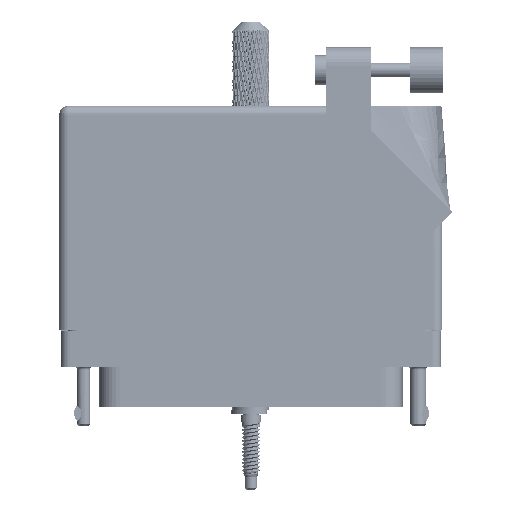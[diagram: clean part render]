
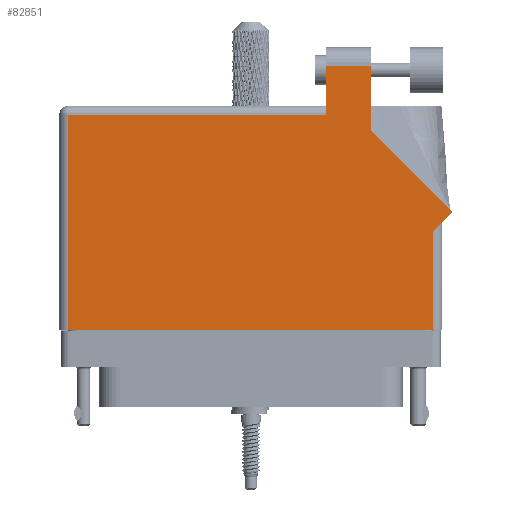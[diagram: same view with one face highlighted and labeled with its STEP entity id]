
A CAD part, front view. The second image highlights one B-rep face of the part: STEP entity #82851.
In plain terms, the highlighted face is planar.
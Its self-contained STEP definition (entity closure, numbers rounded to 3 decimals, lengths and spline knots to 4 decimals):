
#485 = EDGE_LOOP ( 'NONE', ( #99890, #19792, #51032, #76020, #92386, #72344, #46779, #94173, #6920 ) ) ;
#732 = EDGE_CURVE ( 'NONE', #107216, #65128, #65377, .T. ) ;
#1587 = VERTEX_POINT ( 'NONE', #102448 ) ;
#4742 = CARTESIAN_POINT ( 'NONE',  ( 0.82, 1.705, 0.455 ) ) ;
#5393 = LINE ( 'NONE', #80090, #112568 ) ;
#5544 = PLANE ( 'NONE',  #17887 ) ;
#5785 = VERTEX_POINT ( 'NONE', #7285 ) ;
#6920 = ORIENTED_EDGE ( 'NONE', *, *, #72758, .T. ) ;
#7285 = CARTESIAN_POINT ( 'NONE',  ( -1.244, 1.368, 0.455 ) ) ;
#10316 = EDGE_CURVE ( 'NONE', #88586, #28034, #113640, .T. ) ;
#12041 = CARTESIAN_POINT ( 'NONE',  ( 0.513, 1.705, 0.455 ) ) ;
#12218 = DIRECTION ( 'NONE',  ( -1., 0., 0. ) ) ;
#15439 = DIRECTION ( 'NONE',  ( 0., 0., -1. ) ) ;
#17887 = AXIS2_PLACEMENT_3D ( 'NONE', #83074, #15439, #24454 ) ;
#19792 = ORIENTED_EDGE ( 'NONE', *, *, #10316, .T. ) ;
#19816 = VERTEX_POINT ( 'NONE', #70846 ) ;
#22688 = EDGE_CURVE ( 'NONE', #5785, #1587, #123939, .T. ) ;
#24454 = DIRECTION ( 'NONE',  ( -1., 0., 0. ) ) ;
#25063 = VECTOR ( 'NONE', #116954, 39.3701 ) ;
#25431 = VECTOR ( 'NONE', #64995, 39.3701 ) ;
#28034 = VERTEX_POINT ( 'NONE', #12041 ) ;
#30791 = EDGE_CURVE ( 'NONE', #28034, #55289, #57163, .T. ) ;
#33926 = VERTEX_POINT ( 'NONE', #59800 ) ;
#36199 = CARTESIAN_POINT ( 'NONE',  ( 0.513, 1.368, 0.455 ) ) ;
#40316 = DIRECTION ( 'NONE',  ( 0., -1., 0. ) ) ;
#41165 = CARTESIAN_POINT ( 'NONE',  ( -1.244, -0.1, 0.455 ) ) ;
#42579 = CARTESIAN_POINT ( 'NONE',  ( 1.306, 0.637, 0.455 ) ) ;
#42773 = DIRECTION ( 'NONE',  ( -0.707, 0.707, 0. ) ) ;
#43637 = EDGE_CURVE ( 'NONE', #19816, #88586, #93725, .T. ) ;
#46779 = ORIENTED_EDGE ( 'NONE', *, *, #124833, .T. ) ;
#48287 = LINE ( 'NONE', #95018, #25431 ) ;
#48577 = VECTOR ( 'NONE', #42773, 39.3701 ) ;
#48821 = EDGE_CURVE ( 'NONE', #1587, #33926, #48287, .T. ) ;
#50016 = VECTOR ( 'NONE', #102150, 39.3701 ) ;
#51032 = ORIENTED_EDGE ( 'NONE', *, *, #30791, .T. ) ;
#55289 = VERTEX_POINT ( 'NONE', #36199 ) ;
#57163 = LINE ( 'NONE', #106241, #25063 ) ;
#59196 = FACE_OUTER_BOUND ( 'NONE', #485, .T. ) ;
#59800 = CARTESIAN_POINT ( 'NONE',  ( 1.244, -0.1, 0.455 ) ) ;
#60459 = CARTESIAN_POINT ( 'NONE',  ( 1.244, 0.637, 0.455 ) ) ;
#64995 = DIRECTION ( 'NONE',  ( 1., 0., 0. ) ) ;
#65128 = VERTEX_POINT ( 'NONE', #100165 ) ;
#65377 = LINE ( 'NONE', #42579, #50016 ) ;
#67576 = VECTOR ( 'NONE', #100812, 39.3701 ) ;
#67942 = LINE ( 'NONE', #60459, #95517 ) ;
#69182 = VECTOR ( 'NONE', #12218, 39.3701 ) ;
#70343 = VECTOR ( 'NONE', #40316, 39.3701 ) ;
#70846 = CARTESIAN_POINT ( 'NONE',  ( 0.82, 1.2644, 0.455 ) ) ;
#72344 = ORIENTED_EDGE ( 'NONE', *, *, #48821, .T. ) ;
#72758 = EDGE_CURVE ( 'NONE', #65128, #19816, #108417, .T. ) ;
#76020 = ORIENTED_EDGE ( 'NONE', *, *, #93577, .T. ) ;
#80090 = CARTESIAN_POINT ( 'NONE',  ( -1.306, 1.368, 0.455 ) ) ;
#80274 = CARTESIAN_POINT ( 'NONE',  ( 0.82, 1.2644, 0.455 ) ) ;
#81748 = CARTESIAN_POINT ( 'NONE',  ( 1.3767, 0.7077, 0.455 ) ) ;
#82851 = ADVANCED_FACE ( 'NONE', ( #59196 ), #5544, .F. ) ;
#83074 = CARTESIAN_POINT ( 'NONE',  ( -1.306, 1.43, 0.455 ) ) ;
#88586 = VERTEX_POINT ( 'NONE', #4742 ) ;
#89925 = DIRECTION ( 'NONE',  ( -1., 0., 0. ) ) ;
#91035 = CARTESIAN_POINT ( 'NONE',  ( 0.513, 1.705, 0.455 ) ) ;
#92386 = ORIENTED_EDGE ( 'NONE', *, *, #22688, .T. ) ;
#93577 = EDGE_CURVE ( 'NONE', #55289, #5785, #5393, .T. ) ;
#93725 = LINE ( 'NONE', #80274, #67576 ) ;
#94173 = ORIENTED_EDGE ( 'NONE', *, *, #732, .T. ) ;
#95018 = CARTESIAN_POINT ( 'NONE',  ( -1.306, -0.1, 0.455 ) ) ;
#95517 = VECTOR ( 'NONE', #110522, 39.3701 ) ;
#97717 = CARTESIAN_POINT ( 'NONE',  ( 1.244, 0.575, 0.455 ) ) ;
#99890 = ORIENTED_EDGE ( 'NONE', *, *, #43637, .T. ) ;
#100165 = CARTESIAN_POINT ( 'NONE',  ( 1.3767, 0.7077, 0.455 ) ) ;
#100812 = DIRECTION ( 'NONE',  ( 0., 1., 0. ) ) ;
#102150 = DIRECTION ( 'NONE',  ( 0.707, 0.707, 0. ) ) ;
#102448 = CARTESIAN_POINT ( 'NONE',  ( -1.244, -0.1, 0.455 ) ) ;
#106241 = CARTESIAN_POINT ( 'NONE',  ( 0.513, 1.43, 0.455 ) ) ;
#107216 = VERTEX_POINT ( 'NONE', #97717 ) ;
#108417 = LINE ( 'NONE', #81748, #48577 ) ;
#110522 = DIRECTION ( 'NONE',  ( 0., 1., 0. ) ) ;
#112568 = VECTOR ( 'NONE', #89925, 39.3701 ) ;
#113640 = LINE ( 'NONE', #91035, #69182 ) ;
#116954 = DIRECTION ( 'NONE',  ( 0., -1., 0. ) ) ;
#123939 = LINE ( 'NONE', #41165, #70343 ) ;
#124833 = EDGE_CURVE ( 'NONE', #33926, #107216, #67942, .T. ) ;
